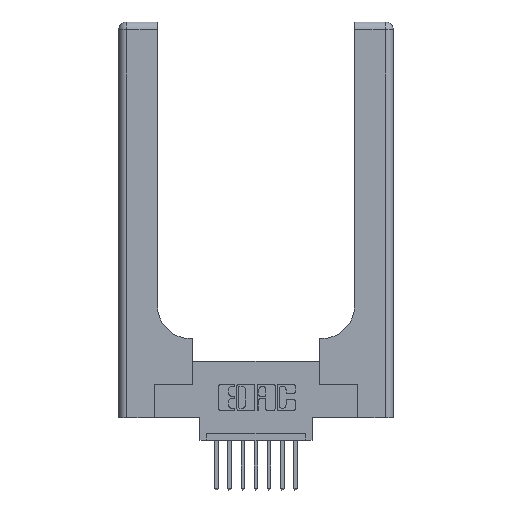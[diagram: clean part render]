
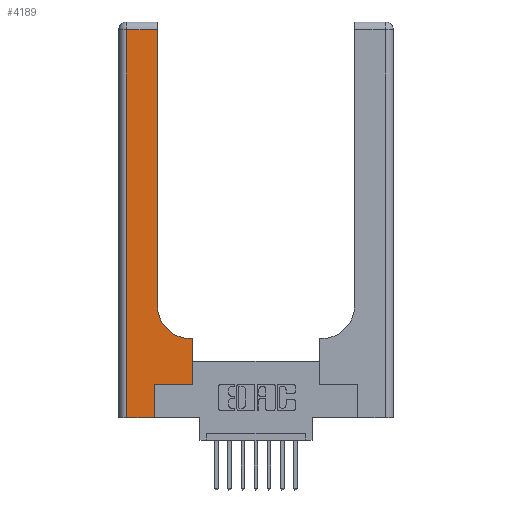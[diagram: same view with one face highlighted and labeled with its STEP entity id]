
A CAD part, top view. The second image highlights one B-rep face of the part: STEP entity #4189.
In plain terms, the highlighted planar face has unit normal (0, 0, 1).
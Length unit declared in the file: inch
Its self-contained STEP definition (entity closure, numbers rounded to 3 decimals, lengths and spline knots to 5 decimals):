
#26 = LINE ( 'NONE', #3120, #10212 ) ;
#594 = VECTOR ( 'NONE', #1654, 39.37008 ) ;
#713 = EDGE_CURVE ( 'NONE', #4241, #975, #1162, .T. ) ;
#927 = DIRECTION ( 'NONE',  ( -1., 0., 0. ) ) ;
#975 = VERTEX_POINT ( 'NONE', #4684 ) ;
#1162 = LINE ( 'NONE', #9983, #594 ) ;
#1276 = CARTESIAN_POINT ( 'NONE',  ( 0.06, 2.94, 0.37 ) ) ;
#1400 = CARTESIAN_POINT ( 'NONE',  ( 0.269, 0., 0.37 ) ) ;
#1455 = ORIENTED_EDGE ( 'NONE', *, *, #3145, .T. ) ;
#1544 = DIRECTION ( 'NONE',  ( -1., 0., 0. ) ) ;
#1654 = DIRECTION ( 'NONE',  ( 1., 0., 0. ) ) ;
#1683 = CARTESIAN_POINT ( 'NONE',  ( 0.5415, 0.85, 0.37 ) ) ;
#1876 = ORIENTED_EDGE ( 'NONE', *, *, #6950, .T. ) ;
#2079 = DIRECTION ( 'NONE',  ( 1., 0., 0. ) ) ;
#2121 = ORIENTED_EDGE ( 'NONE', *, *, #9609, .T. ) ;
#2430 = CARTESIAN_POINT ( 'NONE',  ( 0.06, 0., 0.37 ) ) ;
#2712 = ORIENTED_EDGE ( 'NONE', *, *, #11028, .T. ) ;
#3120 = CARTESIAN_POINT ( 'NONE',  ( 0.2915, 0.6, 0.37 ) ) ;
#3122 = VERTEX_POINT ( 'NONE', #1276 ) ;
#3144 = CARTESIAN_POINT ( 'NONE',  ( 0., 2.94, 0.37 ) ) ;
#3145 = EDGE_CURVE ( 'NONE', #975, #13600, #13076, .T. ) ;
#3495 = ORIENTED_EDGE ( 'NONE', *, *, #713, .T. ) ;
#3522 = VECTOR ( 'NONE', #9688, 39.37008 ) ;
#3573 = ORIENTED_EDGE ( 'NONE', *, *, #15000, .T. ) ;
#3660 = CARTESIAN_POINT ( 'NONE',  ( 0.2915, 0.85, 0.37 ) ) ;
#3949 = CARTESIAN_POINT ( 'NONE',  ( 0.2915, 3., 0.37 ) ) ;
#4189 = ADVANCED_FACE ( 'NONE', ( #4579 ), #12097, .F. ) ;
#4241 = VERTEX_POINT ( 'NONE', #11888 ) ;
#4445 = VERTEX_POINT ( 'NONE', #2430 ) ;
#4578 = EDGE_LOOP ( 'NONE', ( #5160, #2712, #12943, #5365, #2121, #3495, #1455, #1876, #3573 ) ) ;
#4579 = FACE_OUTER_BOUND ( 'NONE', #4578, .T. ) ;
#4684 = CARTESIAN_POINT ( 'NONE',  ( 0.5585, 0.25, 0.37 ) ) ;
#4899 = CARTESIAN_POINT ( 'NONE',  ( 0., 3., 0.37 ) ) ;
#5160 = ORIENTED_EDGE ( 'NONE', *, *, #8458, .T. ) ;
#5257 = DIRECTION ( 'NONE',  ( 1., 0., 0. ) ) ;
#5365 = ORIENTED_EDGE ( 'NONE', *, *, #14072, .T. ) ;
#5461 = DIRECTION ( 'NONE',  ( 0., 0., -1. ) ) ;
#5600 = VECTOR ( 'NONE', #8880, 39.37008 ) ;
#6088 = VERTEX_POINT ( 'NONE', #9164 ) ;
#6210 = VECTOR ( 'NONE', #12913, 39.37008 ) ;
#6619 = VECTOR ( 'NONE', #927, 39.37008 ) ;
#6733 = CARTESIAN_POINT ( 'NONE',  ( 0.5585, 0.6, 0.37 ) ) ;
#6950 = EDGE_CURVE ( 'NONE', #13600, #7866, #26, .T. ) ;
#7461 = VECTOR ( 'NONE', #2079, 39.37008 ) ;
#7812 = AXIS2_PLACEMENT_3D ( 'NONE', #1683, #5461, #5257 ) ;
#7866 = VERTEX_POINT ( 'NONE', #13772 ) ;
#8152 = VERTEX_POINT ( 'NONE', #3660 ) ;
#8388 = AXIS2_PLACEMENT_3D ( 'NONE', #4899, #12046, #1544 ) ;
#8458 = EDGE_CURVE ( 'NONE', #8152, #10145, #8686, .T. ) ;
#8686 = LINE ( 'NONE', #3949, #5600 ) ;
#8880 = DIRECTION ( 'NONE',  ( 0., 1., 0. ) ) ;
#9024 = VECTOR ( 'NONE', #13740, 39.37008 ) ;
#9043 = LINE ( 'NONE', #1400, #3522 ) ;
#9124 = CARTESIAN_POINT ( 'NONE',  ( 0., 0., 0.37 ) ) ;
#9164 = CARTESIAN_POINT ( 'NONE',  ( 0.269, 0., 0.37 ) ) ;
#9511 = LINE ( 'NONE', #13995, #6210 ) ;
#9609 = EDGE_CURVE ( 'NONE', #6088, #4241, #9043, .T. ) ;
#9688 = DIRECTION ( 'NONE',  ( 0., 1., 0. ) ) ;
#9983 = CARTESIAN_POINT ( 'NONE',  ( 0.269, 0.25, 0.37 ) ) ;
#10145 = VERTEX_POINT ( 'NONE', #14617 ) ;
#10212 = VECTOR ( 'NONE', #10375, 39.37008 ) ;
#10375 = DIRECTION ( 'NONE',  ( -1., 0., 0. ) ) ;
#11028 = EDGE_CURVE ( 'NONE', #10145, #3122, #11774, .T. ) ;
#11774 = LINE ( 'NONE', #3144, #6619 ) ;
#11888 = CARTESIAN_POINT ( 'NONE',  ( 0.269, 0.25, 0.37 ) ) ;
#12046 = DIRECTION ( 'NONE',  ( 0., 0., -1. ) ) ;
#12097 = PLANE ( 'NONE',  #8388 ) ;
#12555 = CARTESIAN_POINT ( 'NONE',  ( 0.5585, 0.25, 0.37 ) ) ;
#12913 = DIRECTION ( 'NONE',  ( 0., -1., 0. ) ) ;
#12943 = ORIENTED_EDGE ( 'NONE', *, *, #13181, .T. ) ;
#13076 = LINE ( 'NONE', #12555, #9024 ) ;
#13181 = EDGE_CURVE ( 'NONE', #3122, #4445, #9511, .T. ) ;
#13600 = VERTEX_POINT ( 'NONE', #6733 ) ;
#13740 = DIRECTION ( 'NONE',  ( 0., 1., 0. ) ) ;
#13772 = CARTESIAN_POINT ( 'NONE',  ( 0.5415, 0.6, 0.37 ) ) ;
#13995 = CARTESIAN_POINT ( 'NONE',  ( 0.06, 3., 0.37 ) ) ;
#14072 = EDGE_CURVE ( 'NONE', #4445, #6088, #15191, .T. ) ;
#14617 = CARTESIAN_POINT ( 'NONE',  ( 0.2915, 2.94, 0.37 ) ) ;
#14782 = CIRCLE ( 'NONE', #7812, 0.25 ) ;
#15000 = EDGE_CURVE ( 'NONE', #7866, #8152, #14782, .T. ) ;
#15191 = LINE ( 'NONE', #9124, #7461 ) ;
